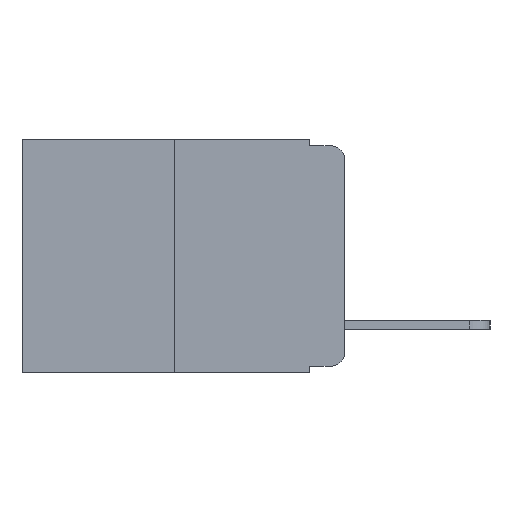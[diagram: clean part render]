
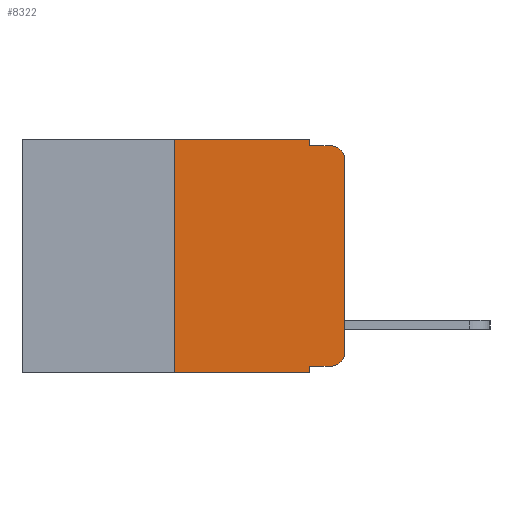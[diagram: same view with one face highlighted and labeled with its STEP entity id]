
A CAD part, left-side view. The second image highlights one B-rep face of the part: STEP entity #8322.
In plain terms, the highlighted planar face has unit normal (-1, 0, 0).
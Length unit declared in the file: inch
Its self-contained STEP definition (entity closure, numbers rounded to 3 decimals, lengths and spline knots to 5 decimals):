
#12 = CARTESIAN_POINT ( 'NONE',  ( 0., 0.473, 0. ) ) ;
#48 = DIRECTION ( 'NONE',  ( 1., 0., 0. ) ) ;
#244 = VECTOR ( 'NONE', #3416, 39.37008 ) ;
#261 = ORIENTED_EDGE ( 'NONE', *, *, #10713, .T. ) ;
#268 = CIRCLE ( 'NONE', #3578, 0.02 ) ;
#324 = EDGE_CURVE ( 'NONE', #692, #10910, #1301, .T. ) ;
#333 = ORIENTED_EDGE ( 'NONE', *, *, #5177, .F. ) ;
#451 = CARTESIAN_POINT ( 'NONE',  ( 0., 0.051, -0.333 ) ) ;
#692 = VERTEX_POINT ( 'NONE', #451 ) ;
#733 = VECTOR ( 'NONE', #8894, 39.37008 ) ;
#745 = DIRECTION ( 'NONE',  ( -1., 0., 0. ) ) ;
#781 = CARTESIAN_POINT ( 'NONE',  ( 0., 0.02, -0.313 ) ) ;
#800 = ORIENTED_EDGE ( 'NONE', *, *, #6940, .F. ) ;
#944 = VERTEX_POINT ( 'NONE', #10482 ) ;
#946 = CARTESIAN_POINT ( 'NONE',  ( 0., 0.25, 0. ) ) ;
#1238 = LINE ( 'NONE', #10903, #4393 ) ;
#1301 = LINE ( 'NONE', #10907, #3227 ) ;
#2387 = VERTEX_POINT ( 'NONE', #2737 ) ;
#2495 = VERTEX_POINT ( 'NONE', #3655 ) ;
#2594 = VERTEX_POINT ( 'NONE', #8755 ) ;
#2604 = CARTESIAN_POINT ( 'NONE',  ( 0., 0.02, -0.333 ) ) ;
#2729 = LINE ( 'NONE', #6534, #4514 ) ;
#2737 = CARTESIAN_POINT ( 'NONE',  ( 0., 0.051, -0.01 ) ) ;
#2746 = LINE ( 'NONE', #7522, #244 ) ;
#2768 = EDGE_CURVE ( 'NONE', #6912, #2387, #7041, .T. ) ;
#2861 = PLANE ( 'NONE',  #9388 ) ;
#2896 = VECTOR ( 'NONE', #4288, 39.37008 ) ;
#2951 = EDGE_CURVE ( 'NONE', #2387, #6095, #1238, .T. ) ;
#3060 = EDGE_CURVE ( 'NONE', #2594, #2495, #6888, .T. ) ;
#3096 = FACE_OUTER_BOUND ( 'NONE', #10751, .T. ) ;
#3227 = VECTOR ( 'NONE', #7393, 39.37008 ) ;
#3333 = EDGE_CURVE ( 'NONE', #692, #9464, #2746, .T. ) ;
#3416 = DIRECTION ( 'NONE',  ( 0., -1., 0. ) ) ;
#3578 = AXIS2_PLACEMENT_3D ( 'NONE', #781, #745, #6965 ) ;
#3620 = LINE ( 'NONE', #12, #733 ) ;
#3655 = CARTESIAN_POINT ( 'NONE',  ( 0., 0., -0.03 ) ) ;
#3685 = DIRECTION ( 'NONE',  ( 0., 0., -1. ) ) ;
#3847 = CARTESIAN_POINT ( 'NONE',  ( 0., 0.02, -0.03 ) ) ;
#4263 = ORIENTED_EDGE ( 'NONE', *, *, #324, .F. ) ;
#4288 = DIRECTION ( 'NONE',  ( 0., 0., -1. ) ) ;
#4393 = VECTOR ( 'NONE', #5584, 39.37008 ) ;
#4463 = CARTESIAN_POINT ( 'NONE',  ( 0., 0.25, 0. ) ) ;
#4514 = VECTOR ( 'NONE', #11021, 39.37008 ) ;
#4542 = CARTESIAN_POINT ( 'NONE',  ( 0., 0.473, 0. ) ) ;
#4935 = CARTESIAN_POINT ( 'NONE',  ( 0., 0.051, -0.343 ) ) ;
#4949 = ORIENTED_EDGE ( 'NONE', *, *, #3060, .T. ) ;
#5177 = EDGE_CURVE ( 'NONE', #944, #10007, #5533, .T. ) ;
#5533 = LINE ( 'NONE', #946, #7915 ) ;
#5584 = DIRECTION ( 'NONE',  ( 0., -1., 0. ) ) ;
#5614 = EDGE_CURVE ( 'NONE', #9464, #2594, #268, .T. ) ;
#5737 = ORIENTED_EDGE ( 'NONE', *, *, #6528, .T. ) ;
#5797 = DIRECTION ( 'NONE',  ( 0., 0., 1. ) ) ;
#6095 = VERTEX_POINT ( 'NONE', #8095 ) ;
#6132 = ORIENTED_EDGE ( 'NONE', *, *, #3333, .T. ) ;
#6276 = CARTESIAN_POINT ( 'NONE',  ( 0., 0.051, 0. ) ) ;
#6528 = EDGE_CURVE ( 'NONE', #944, #10910, #2729, .T. ) ;
#6534 = CARTESIAN_POINT ( 'NONE',  ( 0., 0.473, -0.343 ) ) ;
#6888 = LINE ( 'NONE', #7455, #9657 ) ;
#6912 = VERTEX_POINT ( 'NONE', #6276 ) ;
#6940 = EDGE_CURVE ( 'NONE', #10007, #6912, #3620, .T. ) ;
#6965 = DIRECTION ( 'NONE',  ( 0., 0., -1. ) ) ;
#7041 = LINE ( 'NONE', #9606, #2896 ) ;
#7393 = DIRECTION ( 'NONE',  ( 0., 0., -1. ) ) ;
#7455 = CARTESIAN_POINT ( 'NONE',  ( 0., 0., 0. ) ) ;
#7522 = CARTESIAN_POINT ( 'NONE',  ( 0., 0.051, -0.333 ) ) ;
#7915 = VECTOR ( 'NONE', #10590, 39.37008 ) ;
#8095 = CARTESIAN_POINT ( 'NONE',  ( 0., 0.02, -0.01 ) ) ;
#8263 = DIRECTION ( 'NONE',  ( -1., 0., 0. ) ) ;
#8275 = ORIENTED_EDGE ( 'NONE', *, *, #5614, .T. ) ;
#8322 = ADVANCED_FACE ( 'NONE', ( #3096 ), #2861, .F. ) ;
#8654 = AXIS2_PLACEMENT_3D ( 'NONE', #3847, #8263, #9140 ) ;
#8755 = CARTESIAN_POINT ( 'NONE',  ( 0., 0., -0.313 ) ) ;
#8894 = DIRECTION ( 'NONE',  ( 0., -1., 0. ) ) ;
#9140 = DIRECTION ( 'NONE',  ( 0., 0., -1. ) ) ;
#9388 = AXIS2_PLACEMENT_3D ( 'NONE', #4542, #48, #3685 ) ;
#9464 = VERTEX_POINT ( 'NONE', #2604 ) ;
#9606 = CARTESIAN_POINT ( 'NONE',  ( 0., 0.051, 0. ) ) ;
#9657 = VECTOR ( 'NONE', #5797, 39.37008 ) ;
#9753 = ORIENTED_EDGE ( 'NONE', *, *, #2768, .F. ) ;
#10007 = VERTEX_POINT ( 'NONE', #4463 ) ;
#10482 = CARTESIAN_POINT ( 'NONE',  ( 0., 0.25, -0.343 ) ) ;
#10590 = DIRECTION ( 'NONE',  ( 0., 0., 1. ) ) ;
#10655 = ORIENTED_EDGE ( 'NONE', *, *, #2951, .F. ) ;
#10713 = EDGE_CURVE ( 'NONE', #2495, #6095, #10819, .T. ) ;
#10751 = EDGE_LOOP ( 'NONE', ( #4949, #261, #10655, #9753, #800, #333, #5737, #4263, #6132, #8275 ) ) ;
#10819 = CIRCLE ( 'NONE', #8654, 0.02 ) ;
#10903 = CARTESIAN_POINT ( 'NONE',  ( 0., 0.051, -0.01 ) ) ;
#10907 = CARTESIAN_POINT ( 'NONE',  ( 0., 0.051, 0. ) ) ;
#10910 = VERTEX_POINT ( 'NONE', #4935 ) ;
#11021 = DIRECTION ( 'NONE',  ( 0., -1., 0. ) ) ;
